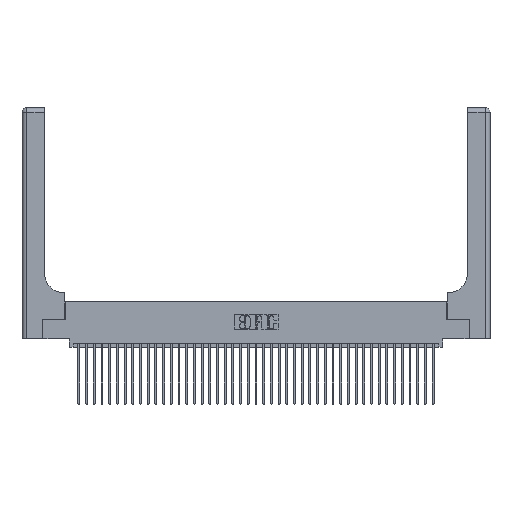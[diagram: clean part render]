
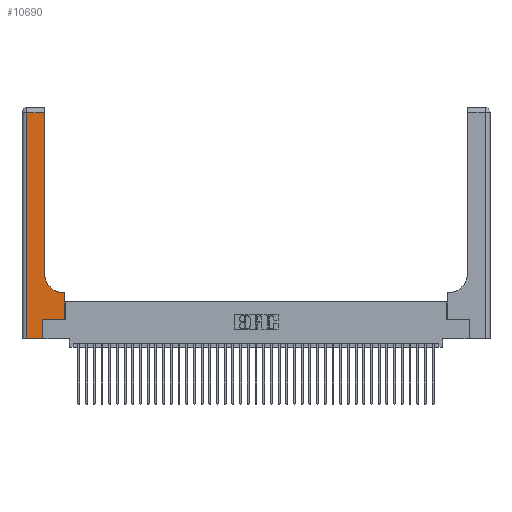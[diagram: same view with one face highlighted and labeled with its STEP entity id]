
A CAD part, top view. The second image highlights one B-rep face of the part: STEP entity #10690.
In plain terms, the highlighted planar face has unit normal (0, 0, 1).
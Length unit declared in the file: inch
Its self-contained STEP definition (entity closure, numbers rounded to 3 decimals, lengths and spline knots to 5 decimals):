
#762 = ORIENTED_EDGE ( 'NONE', *, *, #17036, .T. ) ;
#1115 = CARTESIAN_POINT ( 'NONE',  ( 0.5585, 0.25, 0.37 ) ) ;
#1904 = DIRECTION ( 'NONE',  ( -1., 0., 0. ) ) ;
#2235 = VECTOR ( 'NONE', #2801, 39.37008 ) ;
#2801 = DIRECTION ( 'NONE',  ( 0., -1., 0. ) ) ;
#3110 = CARTESIAN_POINT ( 'NONE',  ( 0.269, 0.25, 0.37 ) ) ;
#3371 = DIRECTION ( 'NONE',  ( -1., 0., 0. ) ) ;
#3925 = CARTESIAN_POINT ( 'NONE',  ( 0.269, 0., 0.37 ) ) ;
#4164 = CARTESIAN_POINT ( 'NONE',  ( 0.5415, 0.6, 0.37 ) ) ;
#4255 = ORIENTED_EDGE ( 'NONE', *, *, #17135, .T. ) ;
#4783 = LINE ( 'NONE', #13010, #11292 ) ;
#5010 = ORIENTED_EDGE ( 'NONE', *, *, #8196, .T. ) ;
#5114 = CARTESIAN_POINT ( 'NONE',  ( 0.2915, 3., 0.37 ) ) ;
#6269 = DIRECTION ( 'NONE',  ( 0., 0., -1. ) ) ;
#6435 = DIRECTION ( 'NONE',  ( 1., 0., 0. ) ) ;
#6909 = VERTEX_POINT ( 'NONE', #23586 ) ;
#7524 = CARTESIAN_POINT ( 'NONE',  ( 0.269, 0.25, 0.37 ) ) ;
#8196 = EDGE_CURVE ( 'NONE', #6909, #8332, #38848, .T. ) ;
#8332 = VERTEX_POINT ( 'NONE', #11806 ) ;
#9461 = CARTESIAN_POINT ( 'NONE',  ( 0.06, 3., 0.37 ) ) ;
#9635 = CARTESIAN_POINT ( 'NONE',  ( 0.2915, 0.85, 0.37 ) ) ;
#10690 = ADVANCED_FACE ( 'NONE', ( #30109 ), #32377, .F. ) ;
#11292 = VECTOR ( 'NONE', #3371, 39.37008 ) ;
#11806 = CARTESIAN_POINT ( 'NONE',  ( 0.06, 0., 0.37 ) ) ;
#11954 = ORIENTED_EDGE ( 'NONE', *, *, #23861, .T. ) ;
#12444 = VERTEX_POINT ( 'NONE', #4164 ) ;
#13010 = CARTESIAN_POINT ( 'NONE',  ( 0., 2.94, 0.37 ) ) ;
#13083 = AXIS2_PLACEMENT_3D ( 'NONE', #25627, #13138, #6435 ) ;
#13138 = DIRECTION ( 'NONE',  ( 0., 0., -1. ) ) ;
#13709 = VECTOR ( 'NONE', #28737, 39.37008 ) ;
#13971 = ORIENTED_EDGE ( 'NONE', *, *, #31087, .T. ) ;
#13977 = CIRCLE ( 'NONE', #13083, 0.25 ) ;
#14259 = VECTOR ( 'NONE', #23113, 39.37008 ) ;
#14711 = CARTESIAN_POINT ( 'NONE',  ( 0.269, 0., 0.37 ) ) ;
#14846 = DIRECTION ( 'NONE',  ( 0., 1., 0. ) ) ;
#16605 = VERTEX_POINT ( 'NONE', #9635 ) ;
#17036 = EDGE_CURVE ( 'NONE', #27143, #38705, #22270, .T. ) ;
#17135 = EDGE_CURVE ( 'NONE', #38705, #39822, #33853, .T. ) ;
#17151 = CARTESIAN_POINT ( 'NONE',  ( 0.2915, 0.6, 0.37 ) ) ;
#18182 = LINE ( 'NONE', #31748, #40322 ) ;
#18331 = VECTOR ( 'NONE', #14846, 39.37008 ) ;
#19192 = CARTESIAN_POINT ( 'NONE',  ( 0.5585, 0.6, 0.37 ) ) ;
#19507 = LINE ( 'NONE', #17151, #37665 ) ;
#19821 = EDGE_CURVE ( 'NONE', #16605, #28064, #39409, .T. ) ;
#20506 = ORIENTED_EDGE ( 'NONE', *, *, #19821, .T. ) ;
#22270 = LINE ( 'NONE', #3110, #13709 ) ;
#23113 = DIRECTION ( 'NONE',  ( 0., 1., 0. ) ) ;
#23586 = CARTESIAN_POINT ( 'NONE',  ( 0.06, 2.94, 0.37 ) ) ;
#23861 = EDGE_CURVE ( 'NONE', #12444, #16605, #13977, .T. ) ;
#23875 = ORIENTED_EDGE ( 'NONE', *, *, #24470, .T. ) ;
#24470 = EDGE_CURVE ( 'NONE', #29489, #27143, #26865, .T. ) ;
#25102 = DIRECTION ( 'NONE',  ( 1., 0., 0. ) ) ;
#25137 = DIRECTION ( 'NONE',  ( 0., 1., 0. ) ) ;
#25448 = CARTESIAN_POINT ( 'NONE',  ( 0., 3., 0.37 ) ) ;
#25595 = CARTESIAN_POINT ( 'NONE',  ( 0.5585, 0.25, 0.37 ) ) ;
#25627 = CARTESIAN_POINT ( 'NONE',  ( 0.5415, 0.85, 0.37 ) ) ;
#26865 = LINE ( 'NONE', #14711, #18331 ) ;
#27143 = VERTEX_POINT ( 'NONE', #7524 ) ;
#27890 = ORIENTED_EDGE ( 'NONE', *, *, #38944, .T. ) ;
#28064 = VERTEX_POINT ( 'NONE', #30907 ) ;
#28737 = DIRECTION ( 'NONE',  ( 1., 0., 0. ) ) ;
#28806 = EDGE_CURVE ( 'NONE', #28064, #6909, #4783, .T. ) ;
#28839 = DIRECTION ( 'NONE',  ( -1., 0., 0. ) ) ;
#29489 = VERTEX_POINT ( 'NONE', #3925 ) ;
#30109 = FACE_OUTER_BOUND ( 'NONE', #36167, .T. ) ;
#30907 = CARTESIAN_POINT ( 'NONE',  ( 0.2915, 2.94, 0.37 ) ) ;
#31087 = EDGE_CURVE ( 'NONE', #8332, #29489, #18182, .T. ) ;
#31748 = CARTESIAN_POINT ( 'NONE',  ( 0., 0., 0.37 ) ) ;
#32377 = PLANE ( 'NONE',  #35542 ) ;
#33853 = LINE ( 'NONE', #1115, #14259 ) ;
#35542 = AXIS2_PLACEMENT_3D ( 'NONE', #25448, #6269, #28839 ) ;
#36167 = EDGE_LOOP ( 'NONE', ( #20506, #41017, #5010, #13971, #23875, #762, #4255, #27890, #11954 ) ) ;
#37665 = VECTOR ( 'NONE', #1904, 39.37008 ) ;
#38705 = VERTEX_POINT ( 'NONE', #25595 ) ;
#38848 = LINE ( 'NONE', #9461, #2235 ) ;
#38944 = EDGE_CURVE ( 'NONE', #39822, #12444, #19507, .T. ) ;
#39409 = LINE ( 'NONE', #5114, #39895 ) ;
#39822 = VERTEX_POINT ( 'NONE', #19192 ) ;
#39895 = VECTOR ( 'NONE', #25137, 39.37008 ) ;
#40322 = VECTOR ( 'NONE', #25102, 39.37008 ) ;
#41017 = ORIENTED_EDGE ( 'NONE', *, *, #28806, .T. ) ;
